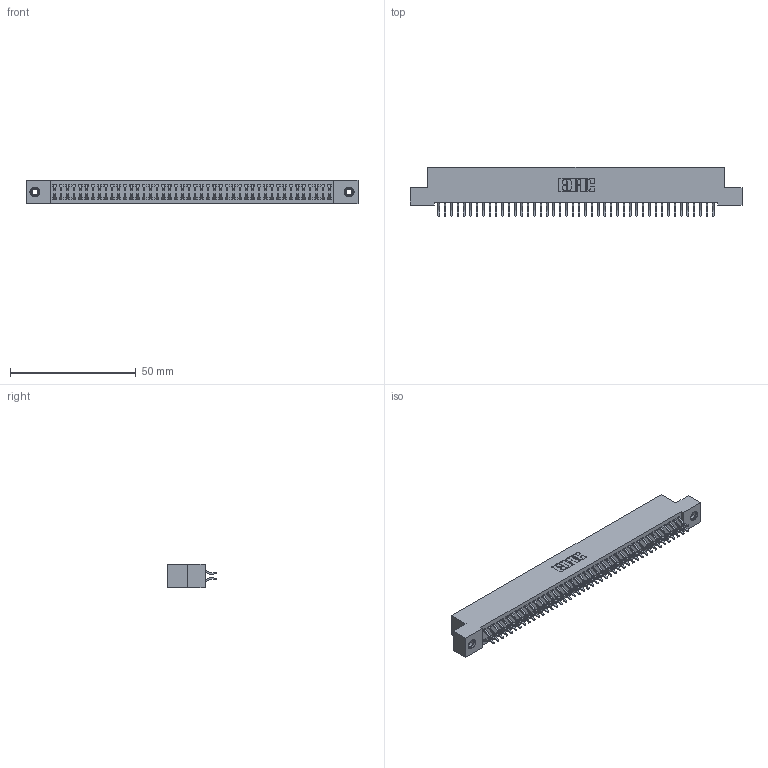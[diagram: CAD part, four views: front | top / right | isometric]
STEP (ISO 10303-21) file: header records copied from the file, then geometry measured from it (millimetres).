
FILE_DESCRIPTION (( 'STEP AP203' ), '1' );
FILE_NAME ('392-088-556-208.STEP', '2019-10-09T17:01:46', ( '' ), ( '' ), 'SwSTEP 2.0', 'SolidWorks 2016', '' );
FILE_SCHEMA (( 'CONFIG_CONTROL_DESIGN' ));
Length unit declared in the file: inch
Products named in the file (4): 392-088-556-208; 342 Part_TI; 345-292-001_556 Tail; 345-250-001_345-250-003-102
Assembly tree (91 placements, depth 2):
  392-088-556-208
    342 Part_TI
    345-292-001_556 Tail  x88
    345-250-001_345-250-003-102  x2
Bounding box: 132.08 x 19.58 x 9.4 mm (x, y, z)
Volume: 11868.9 mm3; surface area: 19293.8 mm2
Topology: 91 solids, 91 shells, 5274 faces, 15659 edges, 10314 vertices
Faces by surface type: plane 3618, cylinder 1640, cone 12, torus 4
Entity records: 29322 total; most frequent: CARTESIAN_POINT 4853, ORIENTED_EDGE 4770, DIRECTION 4163, EDGE_CURVE 2385, VECTOR 2229, LINE 2229, VERTEX_POINT 1584, AXIS2_PLACEMENT_3D 967
